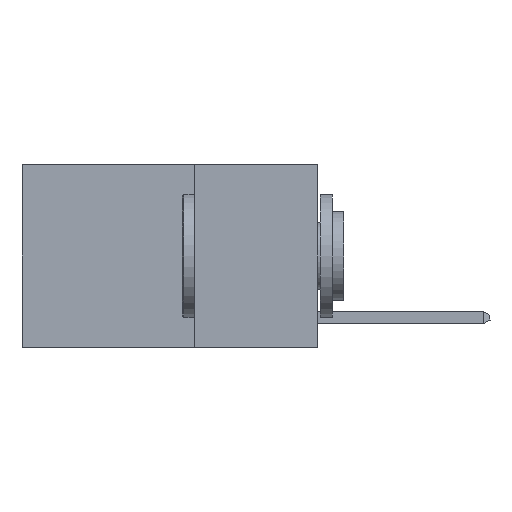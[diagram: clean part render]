
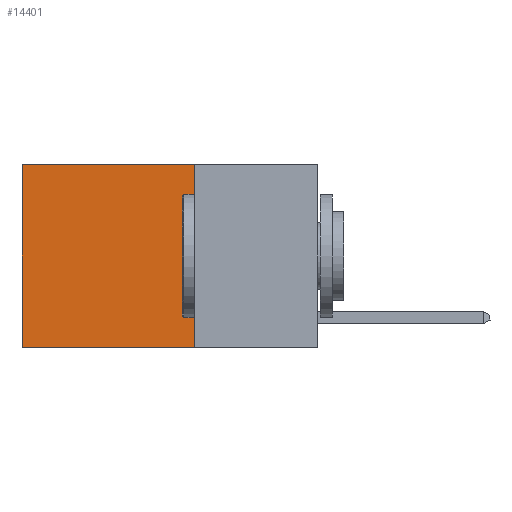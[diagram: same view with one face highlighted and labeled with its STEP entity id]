
A CAD part, left-side view. The second image highlights one B-rep face of the part: STEP entity #14401.
In plain terms, the highlighted planar face has unit normal (-1, 0, 0).
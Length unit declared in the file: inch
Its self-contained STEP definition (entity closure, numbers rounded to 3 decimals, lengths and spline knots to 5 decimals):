
#380 = LINE ( 'NONE', #9950, #18301 ) ;
#923 = VERTEX_POINT ( 'NONE', #1005 ) ;
#1005 = CARTESIAN_POINT ( 'NONE',  ( 0.2625, 0.6, -0.37 ) ) ;
#1361 = DIRECTION ( 'NONE',  ( 0., 0., -1. ) ) ;
#1426 = DIRECTION ( 'NONE',  ( 1., 0., 0. ) ) ;
#1831 = VECTOR ( 'NONE', #18943, 39.37008 ) ;
#2789 = ORIENTED_EDGE ( 'NONE', *, *, #18605, .F. ) ;
#3236 = CARTESIAN_POINT ( 'NONE',  ( 0.2625, 0.25, 0. ) ) ;
#6588 = DIRECTION ( 'NONE',  ( 0., 1., 0. ) ) ;
#7004 = EDGE_CURVE ( 'NONE', #13823, #21039, #11009, .T. ) ;
#7762 = AXIS2_PLACEMENT_3D ( 'NONE', #20388, #1426, #13561 ) ;
#8199 = CARTESIAN_POINT ( 'NONE',  ( 0.2625, 0.25, 0. ) ) ;
#8452 = DIRECTION ( 'NONE',  ( 0., 1., 0. ) ) ;
#9568 = LINE ( 'NONE', #16938, #19297 ) ;
#9950 = CARTESIAN_POINT ( 'NONE',  ( 0.2625, 0.6, 0. ) ) ;
#10037 = EDGE_CURVE ( 'NONE', #13823, #12424, #17597, .T. ) ;
#10682 = ORIENTED_EDGE ( 'NONE', *, *, #7004, .F. ) ;
#11009 = LINE ( 'NONE', #17221, #1831 ) ;
#12424 = VERTEX_POINT ( 'NONE', #18357 ) ;
#13024 = VECTOR ( 'NONE', #8452, 39.37008 ) ;
#13561 = DIRECTION ( 'NONE',  ( 0., 0., -1. ) ) ;
#13823 = VERTEX_POINT ( 'NONE', #8199 ) ;
#14401 = ADVANCED_FACE ( 'NONE', ( #16525 ), #22089, .F. ) ;
#14426 = CARTESIAN_POINT ( 'NONE',  ( 0.2625, 0.25, -0.37 ) ) ;
#15754 = EDGE_LOOP ( 'NONE', ( #18177, #2789, #10682, #18287 ) ) ;
#16525 = FACE_OUTER_BOUND ( 'NONE', #15754, .T. ) ;
#16613 = EDGE_CURVE ( 'NONE', #12424, #923, #380, .T. ) ;
#16938 = CARTESIAN_POINT ( 'NONE',  ( 0.2625, 0.25, -0.37 ) ) ;
#17221 = CARTESIAN_POINT ( 'NONE',  ( 0.2625, 0.25, 0. ) ) ;
#17597 = LINE ( 'NONE', #3236, #13024 ) ;
#18177 = ORIENTED_EDGE ( 'NONE', *, *, #16613, .T. ) ;
#18287 = ORIENTED_EDGE ( 'NONE', *, *, #10037, .T. ) ;
#18301 = VECTOR ( 'NONE', #1361, 39.37008 ) ;
#18357 = CARTESIAN_POINT ( 'NONE',  ( 0.2625, 0.6, 0. ) ) ;
#18605 = EDGE_CURVE ( 'NONE', #21039, #923, #9568, .T. ) ;
#18943 = DIRECTION ( 'NONE',  ( 0., 0., -1. ) ) ;
#19297 = VECTOR ( 'NONE', #6588, 39.37008 ) ;
#20388 = CARTESIAN_POINT ( 'NONE',  ( 0.2625, 0.25, 0. ) ) ;
#21039 = VERTEX_POINT ( 'NONE', #14426 ) ;
#22089 = PLANE ( 'NONE',  #7762 ) ;
